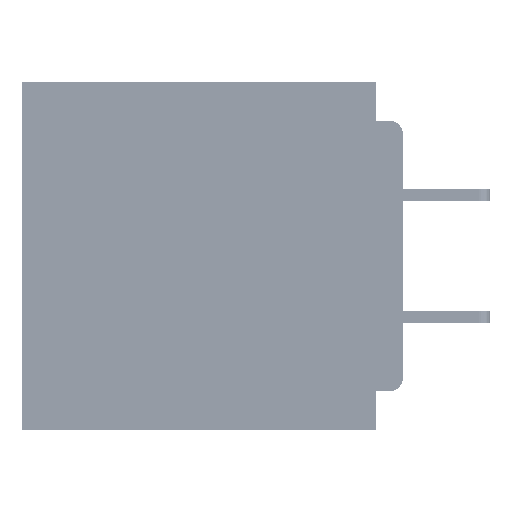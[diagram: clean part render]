
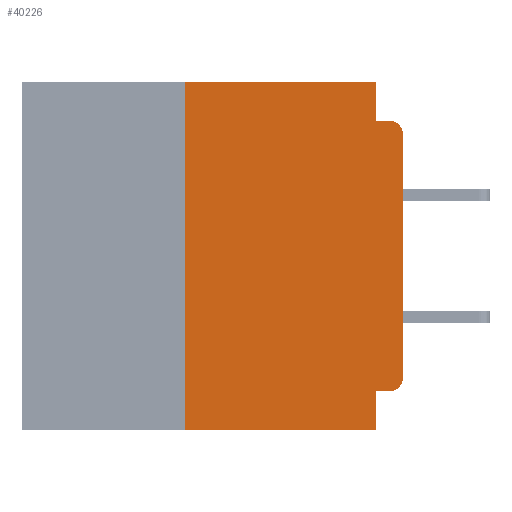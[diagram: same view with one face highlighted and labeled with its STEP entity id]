
A CAD part, left-side view. The second image highlights one B-rep face of the part: STEP entity #40226.
In plain terms, the highlighted planar face has unit normal (-1, 0, 0).
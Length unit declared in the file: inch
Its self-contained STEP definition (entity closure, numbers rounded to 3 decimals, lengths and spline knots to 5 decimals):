
#1291 = CARTESIAN_POINT ( 'NONE',  ( 0., 0.031, 0. ) ) ;
#1651 = DIRECTION ( 'NONE',  ( 0., 0., 1. ) ) ;
#2299 = CARTESIAN_POINT ( 'NONE',  ( 0., 0.015, -0.34 ) ) ;
#2417 = ORIENTED_EDGE ( 'NONE', *, *, #5992, .F. ) ;
#3686 = EDGE_CURVE ( 'NONE', #53612, #65376, #52257, .T. ) ;
#4362 = DIRECTION ( 'NONE',  ( 0., -1., 0. ) ) ;
#5992 = EDGE_CURVE ( 'NONE', #23664, #53938, #48209, .T. ) ;
#6087 = VECTOR ( 'NONE', #29485, 39.37008 ) ;
#6124 = EDGE_CURVE ( 'NONE', #54790, #34941, #13519, .T. ) ;
#7599 = DIRECTION ( 'NONE',  ( 0., 0., -1. ) ) ;
#8034 = DIRECTION ( 'NONE',  ( -1., 0., 0. ) ) ;
#8381 = VECTOR ( 'NONE', #28713, 39.37008 ) ;
#11304 = DIRECTION ( 'NONE',  ( 0., 0., -1. ) ) ;
#12019 = CARTESIAN_POINT ( 'NONE',  ( 0., 0.25, -0.4 ) ) ;
#12099 = PLANE ( 'NONE',  #42368 ) ;
#12519 = CIRCLE ( 'NONE', #31311, 0.015 ) ;
#12834 = CARTESIAN_POINT ( 'NONE',  ( 0., 0.031, -0.355 ) ) ;
#13253 = EDGE_CURVE ( 'NONE', #19731, #40487, #67259, .T. ) ;
#13519 = LINE ( 'NONE', #23741, #52259 ) ;
#14467 = CARTESIAN_POINT ( 'NONE',  ( 0., 0., -0.355 ) ) ;
#17469 = CARTESIAN_POINT ( 'NONE',  ( 0., 0.437, 0. ) ) ;
#17500 = CARTESIAN_POINT ( 'NONE',  ( 0., 0.015, -0.045 ) ) ;
#18584 = CIRCLE ( 'NONE', #39714, 0.015 ) ;
#18860 = CARTESIAN_POINT ( 'NONE',  ( 0., 0., -0.045 ) ) ;
#19148 = LINE ( 'NONE', #1291, #33171 ) ;
#19731 = VERTEX_POINT ( 'NONE', #12019 ) ;
#20215 = CARTESIAN_POINT ( 'NONE',  ( 0., 0., -0.34 ) ) ;
#20542 = VECTOR ( 'NONE', #11304, 39.37008 ) ;
#21231 = ORIENTED_EDGE ( 'NONE', *, *, #13253, .F. ) ;
#22505 = LINE ( 'NONE', #23405, #8381 ) ;
#22809 = DIRECTION ( 'NONE',  ( 1., 0., 0. ) ) ;
#23163 = EDGE_LOOP ( 'NONE', ( #65916, #37528, #2417, #36902, #45130, #21231, #53509, #36087, #62924, #46922 ) ) ;
#23331 = VERTEX_POINT ( 'NONE', #53913 ) ;
#23405 = CARTESIAN_POINT ( 'NONE',  ( 0., 0.437, 0. ) ) ;
#23441 = EDGE_CURVE ( 'NONE', #53612, #54790, #12519, .T. ) ;
#23664 = VERTEX_POINT ( 'NONE', #40883 ) ;
#23741 = CARTESIAN_POINT ( 'NONE',  ( 0., 0., 0. ) ) ;
#23761 = EDGE_CURVE ( 'NONE', #44447, #23664, #19148, .T. ) ;
#28047 = CARTESIAN_POINT ( 'NONE',  ( 0., 0.25, -0.4 ) ) ;
#28713 = DIRECTION ( 'NONE',  ( 0., -1., 0. ) ) ;
#29485 = DIRECTION ( 'NONE',  ( 0., -1., 0. ) ) ;
#31311 = AXIS2_PLACEMENT_3D ( 'NONE', #2299, #39276, #7599 ) ;
#33171 = VECTOR ( 'NONE', #38241, 39.37008 ) ;
#34941 = VERTEX_POINT ( 'NONE', #43118 ) ;
#36087 = ORIENTED_EDGE ( 'NONE', *, *, #43337, .F. ) ;
#36206 = LINE ( 'NONE', #53474, #20542 ) ;
#36902 = ORIENTED_EDGE ( 'NONE', *, *, #23761, .F. ) ;
#37528 = ORIENTED_EDGE ( 'NONE', *, *, #37700, .T. ) ;
#37700 = EDGE_CURVE ( 'NONE', #34941, #53938, #18584, .T. ) ;
#38241 = DIRECTION ( 'NONE',  ( 0., 0., -1. ) ) ;
#38274 = FACE_OUTER_BOUND ( 'NONE', #23163, .T. ) ;
#38315 = VECTOR ( 'NONE', #67002, 39.37008 ) ;
#39162 = EDGE_CURVE ( 'NONE', #40487, #44447, #22505, .T. ) ;
#39276 = DIRECTION ( 'NONE',  ( -1., 0., 0. ) ) ;
#39714 = AXIS2_PLACEMENT_3D ( 'NONE', #39725, #8034, #45019 ) ;
#39725 = CARTESIAN_POINT ( 'NONE',  ( 0., 0.015, -0.06 ) ) ;
#40226 = ADVANCED_FACE ( 'NONE', ( #38274 ), #12099, .F. ) ;
#40487 = VERTEX_POINT ( 'NONE', #50599 ) ;
#40883 = CARTESIAN_POINT ( 'NONE',  ( 0., 0.031, -0.045 ) ) ;
#42368 = AXIS2_PLACEMENT_3D ( 'NONE', #17469, #22809, #59490 ) ;
#43118 = CARTESIAN_POINT ( 'NONE',  ( 0., 0., -0.06 ) ) ;
#43337 = EDGE_CURVE ( 'NONE', #65376, #23331, #36206, .T. ) ;
#44447 = VERTEX_POINT ( 'NONE', #46648 ) ;
#45019 = DIRECTION ( 'NONE',  ( 0., 0., -1. ) ) ;
#45130 = ORIENTED_EDGE ( 'NONE', *, *, #39162, .F. ) ;
#46413 = CARTESIAN_POINT ( 'NONE',  ( 0., 0.437, -0.4 ) ) ;
#46648 = CARTESIAN_POINT ( 'NONE',  ( 0., 0.031, 0. ) ) ;
#46922 = ORIENTED_EDGE ( 'NONE', *, *, #23441, .T. ) ;
#48209 = LINE ( 'NONE', #18860, #6087 ) ;
#48215 = VECTOR ( 'NONE', #4362, 39.37008 ) ;
#49932 = DIRECTION ( 'NONE',  ( 0., 0., 1. ) ) ;
#50599 = CARTESIAN_POINT ( 'NONE',  ( 0., 0.25, 0. ) ) ;
#52257 = LINE ( 'NONE', #14467, #38315 ) ;
#52259 = VECTOR ( 'NONE', #49932, 39.37008 ) ;
#53474 = CARTESIAN_POINT ( 'NONE',  ( 0., 0.031, -0.4 ) ) ;
#53509 = ORIENTED_EDGE ( 'NONE', *, *, #64951, .T. ) ;
#53612 = VERTEX_POINT ( 'NONE', #67039 ) ;
#53913 = CARTESIAN_POINT ( 'NONE',  ( 0., 0.031, -0.4 ) ) ;
#53938 = VERTEX_POINT ( 'NONE', #17500 ) ;
#54790 = VERTEX_POINT ( 'NONE', #20215 ) ;
#55059 = VECTOR ( 'NONE', #1651, 39.37008 ) ;
#59490 = DIRECTION ( 'NONE',  ( 0., 0., -1. ) ) ;
#62924 = ORIENTED_EDGE ( 'NONE', *, *, #3686, .F. ) ;
#63649 = LINE ( 'NONE', #46413, #48215 ) ;
#64951 = EDGE_CURVE ( 'NONE', #19731, #23331, #63649, .T. ) ;
#65376 = VERTEX_POINT ( 'NONE', #12834 ) ;
#65916 = ORIENTED_EDGE ( 'NONE', *, *, #6124, .T. ) ;
#67002 = DIRECTION ( 'NONE',  ( 0., 1., 0. ) ) ;
#67039 = CARTESIAN_POINT ( 'NONE',  ( 0., 0.015, -0.355 ) ) ;
#67259 = LINE ( 'NONE', #28047, #55059 ) ;
